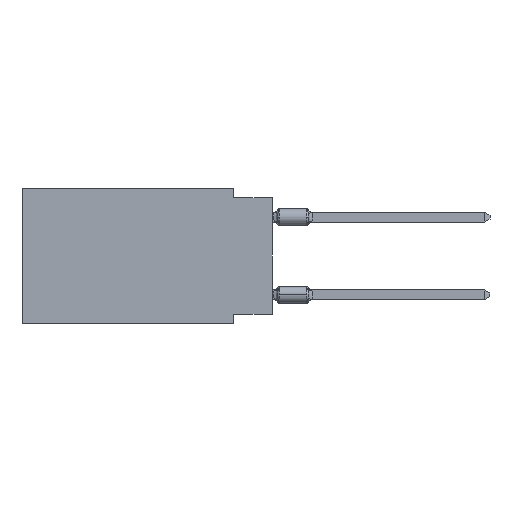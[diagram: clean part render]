
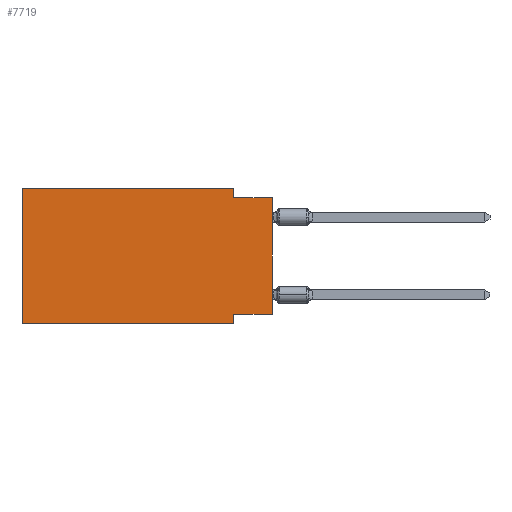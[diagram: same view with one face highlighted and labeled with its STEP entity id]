
A CAD part, left-side view. The second image highlights one B-rep face of the part: STEP entity #7719.
In plain terms, the highlighted planar face has unit normal (-1, 0, 0).
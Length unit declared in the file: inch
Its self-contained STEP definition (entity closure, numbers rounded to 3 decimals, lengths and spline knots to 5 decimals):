
#7 = VERTEX_POINT ( 'NONE', #13421 ) ;
#127 = VERTEX_POINT ( 'NONE', #19895 ) ;
#238 = DIRECTION ( 'NONE',  ( 0., -1., 0. ) ) ;
#710 = AXIS2_PLACEMENT_3D ( 'NONE', #6827, #19165, #18867 ) ;
#1062 = LINE ( 'NONE', #15161, #7944 ) ;
#1151 = VECTOR ( 'NONE', #12202, 39.37008 ) ;
#1188 = EDGE_CURVE ( 'NONE', #9812, #127, #12906, .T. ) ;
#1468 = VERTEX_POINT ( 'NONE', #6131 ) ;
#1905 = VECTOR ( 'NONE', #17734, 39.37008 ) ;
#2169 = CARTESIAN_POINT ( 'NONE',  ( 0., 0.1, -0.35 ) ) ;
#2336 = VECTOR ( 'NONE', #18852, 39.37008 ) ;
#2919 = EDGE_CURVE ( 'NONE', #19402, #3979, #15600, .T. ) ;
#3113 = CARTESIAN_POINT ( 'NONE',  ( 0., 0., -0.025 ) ) ;
#3243 = CARTESIAN_POINT ( 'NONE',  ( 0., 0.645, -0.35 ) ) ;
#3637 = DIRECTION ( 'NONE',  ( 0., 0., 1. ) ) ;
#3764 = CARTESIAN_POINT ( 'NONE',  ( 0., 0., 0. ) ) ;
#3979 = VERTEX_POINT ( 'NONE', #3113 ) ;
#4446 = EDGE_CURVE ( 'NONE', #127, #1468, #5843, .T. ) ;
#4738 = CARTESIAN_POINT ( 'NONE',  ( 0., 0.645, 0. ) ) ;
#4801 = VECTOR ( 'NONE', #9900, 39.37008 ) ;
#5018 = FACE_OUTER_BOUND ( 'NONE', #8610, .T. ) ;
#5155 = ORIENTED_EDGE ( 'NONE', *, *, #2919, .F. ) ;
#5645 = ORIENTED_EDGE ( 'NONE', *, *, #18589, .F. ) ;
#5707 = ORIENTED_EDGE ( 'NONE', *, *, #4446, .F. ) ;
#5843 = LINE ( 'NONE', #4738, #1151 ) ;
#5879 = DIRECTION ( 'NONE',  ( 0., 0., -1. ) ) ;
#5897 = ORIENTED_EDGE ( 'NONE', *, *, #18700, .T. ) ;
#6131 = CARTESIAN_POINT ( 'NONE',  ( 0., 0.1, 0. ) ) ;
#6389 = ORIENTED_EDGE ( 'NONE', *, *, #18113, .F. ) ;
#6827 = CARTESIAN_POINT ( 'NONE',  ( 0., 0.645, 0. ) ) ;
#7719 = ADVANCED_FACE ( 'NONE', ( #5018 ), #17534, .F. ) ;
#7944 = VECTOR ( 'NONE', #5879, 39.37008 ) ;
#8610 = EDGE_LOOP ( 'NONE', ( #13682, #5155, #6389, #5707, #17175, #5897, #18145, #5645 ) ) ;
#8989 = CARTESIAN_POINT ( 'NONE',  ( 0., 0., -0.325 ) ) ;
#9812 = VERTEX_POINT ( 'NONE', #3243 ) ;
#9900 = DIRECTION ( 'NONE',  ( 0., 0., 1. ) ) ;
#11262 = CARTESIAN_POINT ( 'NONE',  ( 0., 0.1, 0. ) ) ;
#11800 = CARTESIAN_POINT ( 'NONE',  ( 0., 0.1, -0.025 ) ) ;
#11937 = DIRECTION ( 'NONE',  ( 0., 1., 0. ) ) ;
#12202 = DIRECTION ( 'NONE',  ( 0., -1., 0. ) ) ;
#12572 = CARTESIAN_POINT ( 'NONE',  ( 0., 0., -0.025 ) ) ;
#12906 = LINE ( 'NONE', #18984, #19057 ) ;
#13038 = LINE ( 'NONE', #3764, #4801 ) ;
#13421 = CARTESIAN_POINT ( 'NONE',  ( 0., 0., -0.325 ) ) ;
#13643 = LINE ( 'NONE', #8989, #15989 ) ;
#13682 = ORIENTED_EDGE ( 'NONE', *, *, #17933, .T. ) ;
#13904 = CARTESIAN_POINT ( 'NONE',  ( 0., 0.1, -0.325 ) ) ;
#15161 = CARTESIAN_POINT ( 'NONE',  ( 0., 0.1, -0.35 ) ) ;
#15556 = LINE ( 'NONE', #18513, #18610 ) ;
#15600 = LINE ( 'NONE', #12572, #2336 ) ;
#15989 = VECTOR ( 'NONE', #11937, 39.37008 ) ;
#15995 = LINE ( 'NONE', #11262, #1905 ) ;
#16795 = VERTEX_POINT ( 'NONE', #13904 ) ;
#17175 = ORIENTED_EDGE ( 'NONE', *, *, #1188, .F. ) ;
#17534 = PLANE ( 'NONE',  #710 ) ;
#17734 = DIRECTION ( 'NONE',  ( 0., 0., -1. ) ) ;
#17933 = EDGE_CURVE ( 'NONE', #7, #3979, #13038, .T. ) ;
#18113 = EDGE_CURVE ( 'NONE', #1468, #19402, #15995, .T. ) ;
#18145 = ORIENTED_EDGE ( 'NONE', *, *, #18564, .F. ) ;
#18434 = VERTEX_POINT ( 'NONE', #2169 ) ;
#18513 = CARTESIAN_POINT ( 'NONE',  ( 0., 0.645, -0.35 ) ) ;
#18564 = EDGE_CURVE ( 'NONE', #16795, #18434, #1062, .T. ) ;
#18589 = EDGE_CURVE ( 'NONE', #7, #16795, #13643, .T. ) ;
#18610 = VECTOR ( 'NONE', #238, 39.37008 ) ;
#18700 = EDGE_CURVE ( 'NONE', #9812, #18434, #15556, .T. ) ;
#18852 = DIRECTION ( 'NONE',  ( 0., -1., 0. ) ) ;
#18867 = DIRECTION ( 'NONE',  ( 0., 0., -1. ) ) ;
#18984 = CARTESIAN_POINT ( 'NONE',  ( 0., 0.645, 0. ) ) ;
#19057 = VECTOR ( 'NONE', #3637, 39.37008 ) ;
#19165 = DIRECTION ( 'NONE',  ( 1., 0., 0. ) ) ;
#19402 = VERTEX_POINT ( 'NONE', #11800 ) ;
#19895 = CARTESIAN_POINT ( 'NONE',  ( 0., 0.645, 0. ) ) ;
